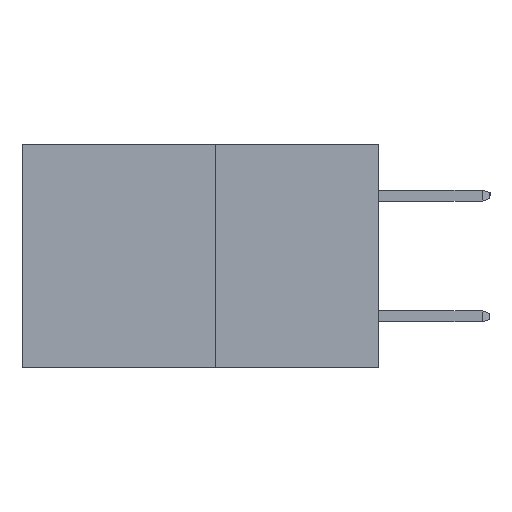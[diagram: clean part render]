
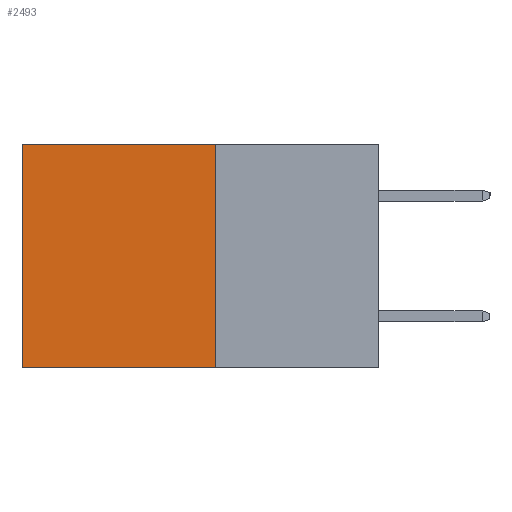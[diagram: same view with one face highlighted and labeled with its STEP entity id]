
A CAD part, left-side view. The second image highlights one B-rep face of the part: STEP entity #2493.
In plain terms, the highlighted planar face has unit normal (-1, 0, 0).
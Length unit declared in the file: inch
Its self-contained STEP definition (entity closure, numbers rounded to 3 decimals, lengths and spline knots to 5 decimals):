
#123 = DIRECTION ( 'NONE',  ( 0., 1., 0. ) ) ;
#128 = EDGE_CURVE ( 'NONE', #9517, #2650, #7992, .T. ) ;
#587 = VECTOR ( 'NONE', #736, 39.37008 ) ;
#736 = DIRECTION ( 'NONE',  ( 0., 0., -1. ) ) ;
#1018 = EDGE_CURVE ( 'NONE', #1098, #2650, #2425, .T. ) ;
#1098 = VERTEX_POINT ( 'NONE', #7837 ) ;
#1116 = EDGE_CURVE ( 'NONE', #8146, #1098, #5831, .T. ) ;
#1216 = CARTESIAN_POINT ( 'NONE',  ( 0.277, 0.27, 0. ) ) ;
#1270 = ORIENTED_EDGE ( 'NONE', *, *, #1116, .T. ) ;
#1336 = VECTOR ( 'NONE', #6014, 39.37008 ) ;
#1883 = VECTOR ( 'NONE', #123, 39.37008 ) ;
#2387 = DIRECTION ( 'NONE',  ( 0., 0., -1. ) ) ;
#2425 = LINE ( 'NONE', #9187, #6625 ) ;
#2493 = ADVANCED_FACE ( 'NONE', ( #6475 ), #10459, .F. ) ;
#2650 = VERTEX_POINT ( 'NONE', #8076 ) ;
#2864 = EDGE_LOOP ( 'NONE', ( #9392, #6574, #5637, #1270 ) ) ;
#3545 = CARTESIAN_POINT ( 'NONE',  ( 0.277, 0.27, -0.37 ) ) ;
#5637 = ORIENTED_EDGE ( 'NONE', *, *, #10052, .F. ) ;
#5831 = LINE ( 'NONE', #1216, #1883 ) ;
#6014 = DIRECTION ( 'NONE',  ( 0., 1., 0. ) ) ;
#6475 = FACE_OUTER_BOUND ( 'NONE', #2864, .T. ) ;
#6574 = ORIENTED_EDGE ( 'NONE', *, *, #128, .F. ) ;
#6625 = VECTOR ( 'NONE', #2387, 39.37008 ) ;
#6690 = CARTESIAN_POINT ( 'NONE',  ( 0.277, 0.27, 0. ) ) ;
#6826 = CARTESIAN_POINT ( 'NONE',  ( 0.277, 0.27, -0.37 ) ) ;
#6992 = AXIS2_PLACEMENT_3D ( 'NONE', #10649, #10421, #10361 ) ;
#7352 = LINE ( 'NONE', #10588, #587 ) ;
#7837 = CARTESIAN_POINT ( 'NONE',  ( 0.277, 0.59, 0. ) ) ;
#7992 = LINE ( 'NONE', #3545, #1336 ) ;
#8076 = CARTESIAN_POINT ( 'NONE',  ( 0.277, 0.59, -0.37 ) ) ;
#8146 = VERTEX_POINT ( 'NONE', #6690 ) ;
#9187 = CARTESIAN_POINT ( 'NONE',  ( 0.277, 0.59, -0.37 ) ) ;
#9392 = ORIENTED_EDGE ( 'NONE', *, *, #1018, .T. ) ;
#9517 = VERTEX_POINT ( 'NONE', #6826 ) ;
#10052 = EDGE_CURVE ( 'NONE', #8146, #9517, #7352, .T. ) ;
#10361 = DIRECTION ( 'NONE',  ( 0., 0., -1. ) ) ;
#10421 = DIRECTION ( 'NONE',  ( 1., 0., 0. ) ) ;
#10459 = PLANE ( 'NONE',  #6992 ) ;
#10588 = CARTESIAN_POINT ( 'NONE',  ( 0.277, 0.27, -0.37 ) ) ;
#10649 = CARTESIAN_POINT ( 'NONE',  ( 0.277, 0.27, -0.37 ) ) ;
